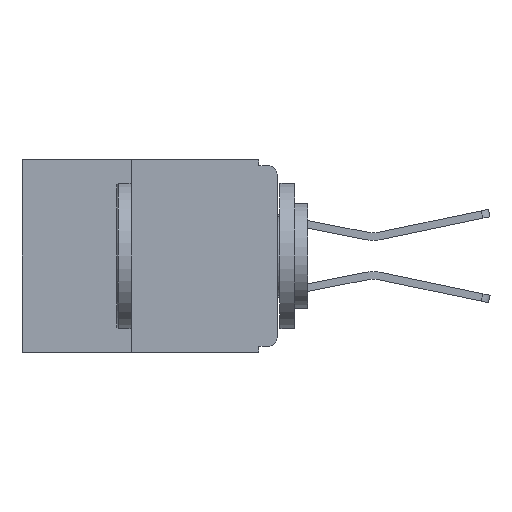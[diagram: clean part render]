
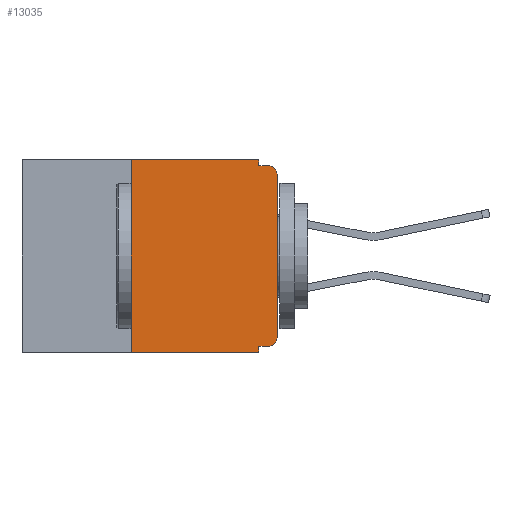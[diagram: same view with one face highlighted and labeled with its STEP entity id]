
A CAD part, left-side view. The second image highlights one B-rep face of the part: STEP entity #13035.
In plain terms, the highlighted planar face has unit normal (-1, 0, 0).
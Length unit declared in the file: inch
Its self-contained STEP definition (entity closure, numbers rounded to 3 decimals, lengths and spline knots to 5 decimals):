
#142 = LINE ( 'NONE', #11878, #17876 ) ;
#284 = PLANE ( 'NONE',  #6104 ) ;
#497 = LINE ( 'NONE', #16744, #20799 ) ;
#806 = VECTOR ( 'NONE', #19617, 39.37008 ) ;
#1842 = EDGE_CURVE ( 'NONE', #16972, #13826, #2128, .T. ) ;
#2007 = DIRECTION ( 'NONE',  ( 0., 1., 0. ) ) ;
#2038 = DIRECTION ( 'NONE',  ( 0., 0., -1. ) ) ;
#2128 = CIRCLE ( 'NONE', #12743, 0.015 ) ;
#2918 = CARTESIAN_POINT ( 'NONE',  ( 0., 0.437, -0.33 ) ) ;
#3091 = EDGE_LOOP ( 'NONE', ( #5953, #6841, #7279, #8026, #8221, #8850, #8959, #9410, #9436, #9678 ) ) ;
#3708 = EDGE_CURVE ( 'NONE', #13333, #16972, #19767, .T. ) ;
#3955 = FACE_OUTER_BOUND ( 'NONE', #3091, .T. ) ;
#4401 = VECTOR ( 'NONE', #7815, 39.37008 ) ;
#5539 = LINE ( 'NONE', #18326, #6081 ) ;
#5917 = EDGE_CURVE ( 'NONE', #13370, #14967, #497, .T. ) ;
#5953 = ORIENTED_EDGE ( 'NONE', *, *, #3708, .T. ) ;
#6081 = VECTOR ( 'NONE', #7314, 39.37008 ) ;
#6104 = AXIS2_PLACEMENT_3D ( 'NONE', #7017, #11906, #2038 ) ;
#6739 = CARTESIAN_POINT ( 'NONE',  ( 0., 0.015, -0.32 ) ) ;
#6783 = CARTESIAN_POINT ( 'NONE',  ( 0., 0.031, 0. ) ) ;
#6839 = CARTESIAN_POINT ( 'NONE',  ( 0., 0.015, -0.305 ) ) ;
#6841 = ORIENTED_EDGE ( 'NONE', *, *, #1842, .T. ) ;
#7017 = CARTESIAN_POINT ( 'NONE',  ( 0., 0.437, 0. ) ) ;
#7279 = ORIENTED_EDGE ( 'NONE', *, *, #15990, .F. ) ;
#7314 = DIRECTION ( 'NONE',  ( 0., 0., 1. ) ) ;
#7450 = EDGE_CURVE ( 'NONE', #12885, #13370, #142, .T. ) ;
#7681 = EDGE_CURVE ( 'NONE', #9169, #18396, #13587, .T. ) ;
#7815 = DIRECTION ( 'NONE',  ( 0., 0., -1. ) ) ;
#8026 = ORIENTED_EDGE ( 'NONE', *, *, #7681, .F. ) ;
#8184 = CARTESIAN_POINT ( 'NONE',  ( 0., 0.031, -0.32 ) ) ;
#8221 = ORIENTED_EDGE ( 'NONE', *, *, #17126, .F. ) ;
#8466 = DIRECTION ( 'NONE',  ( 0., 0., -1. ) ) ;
#8850 = ORIENTED_EDGE ( 'NONE', *, *, #12443, .F. ) ;
#8959 = ORIENTED_EDGE ( 'NONE', *, *, #10276, .T. ) ;
#9169 = VERTEX_POINT ( 'NONE', #6783 ) ;
#9184 = LINE ( 'NONE', #18092, #806 ) ;
#9410 = ORIENTED_EDGE ( 'NONE', *, *, #5917, .F. ) ;
#9436 = ORIENTED_EDGE ( 'NONE', *, *, #7450, .F. ) ;
#9678 = ORIENTED_EDGE ( 'NONE', *, *, #15358, .T. ) ;
#10170 = DIRECTION ( 'NONE',  ( 0., 0., -1. ) ) ;
#10276 = EDGE_CURVE ( 'NONE', #13499, #14967, #13769, .T. ) ;
#11878 = CARTESIAN_POINT ( 'NONE',  ( 0., 0., -0.32 ) ) ;
#11906 = DIRECTION ( 'NONE',  ( 1., 0., 0. ) ) ;
#12387 = VERTEX_POINT ( 'NONE', #13677 ) ;
#12443 = EDGE_CURVE ( 'NONE', #13499, #12387, #5539, .T. ) ;
#12738 = DIRECTION ( 'NONE',  ( 0., -1., 0. ) ) ;
#12743 = AXIS2_PLACEMENT_3D ( 'NONE', #20575, #19091, #10170 ) ;
#12885 = VERTEX_POINT ( 'NONE', #6739 ) ;
#13035 = ADVANCED_FACE ( 'NONE', ( #3955 ), #284, .F. ) ;
#13261 = VECTOR ( 'NONE', #12738, 39.37008 ) ;
#13333 = VERTEX_POINT ( 'NONE', #19001 ) ;
#13370 = VERTEX_POINT ( 'NONE', #8184 ) ;
#13499 = VERTEX_POINT ( 'NONE', #19460 ) ;
#13587 = LINE ( 'NONE', #18803, #4401 ) ;
#13677 = CARTESIAN_POINT ( 'NONE',  ( 0., 0.25, 0. ) ) ;
#13769 = LINE ( 'NONE', #2918, #13261 ) ;
#13826 = VERTEX_POINT ( 'NONE', #18784 ) ;
#14967 = VERTEX_POINT ( 'NONE', #15327 ) ;
#15327 = CARTESIAN_POINT ( 'NONE',  ( 0., 0.031, -0.33 ) ) ;
#15358 = EDGE_CURVE ( 'NONE', #12885, #13333, #16205, .T. ) ;
#15990 = EDGE_CURVE ( 'NONE', #18396, #13826, #16426, .T. ) ;
#16205 = CIRCLE ( 'NONE', #20205, 0.015 ) ;
#16249 = CARTESIAN_POINT ( 'NONE',  ( 0., 0., -0.025 ) ) ;
#16258 = DIRECTION ( 'NONE',  ( 0., 0., 1. ) ) ;
#16359 = CARTESIAN_POINT ( 'NONE',  ( 0., 0., 0. ) ) ;
#16426 = LINE ( 'NONE', #16479, #20436 ) ;
#16479 = CARTESIAN_POINT ( 'NONE',  ( 0., 0., -0.01 ) ) ;
#16682 = DIRECTION ( 'NONE',  ( 0., 0., -1. ) ) ;
#16744 = CARTESIAN_POINT ( 'NONE',  ( 0., 0.031, -0.33 ) ) ;
#16972 = VERTEX_POINT ( 'NONE', #16249 ) ;
#17126 = EDGE_CURVE ( 'NONE', #12387, #9169, #9184, .T. ) ;
#17857 = DIRECTION ( 'NONE',  ( -1., 0., 0. ) ) ;
#17876 = VECTOR ( 'NONE', #2007, 39.37008 ) ;
#18092 = CARTESIAN_POINT ( 'NONE',  ( 0., 0.437, 0. ) ) ;
#18326 = CARTESIAN_POINT ( 'NONE',  ( 0., 0.25, -0.33 ) ) ;
#18396 = VERTEX_POINT ( 'NONE', #19975 ) ;
#18784 = CARTESIAN_POINT ( 'NONE',  ( 0., 0.015, -0.01 ) ) ;
#18803 = CARTESIAN_POINT ( 'NONE',  ( 0., 0.031, 0. ) ) ;
#19001 = CARTESIAN_POINT ( 'NONE',  ( 0., 0., -0.305 ) ) ;
#19091 = DIRECTION ( 'NONE',  ( -1., 0., 0. ) ) ;
#19282 = VECTOR ( 'NONE', #16258, 39.37008 ) ;
#19460 = CARTESIAN_POINT ( 'NONE',  ( 0., 0.25, -0.33 ) ) ;
#19502 = DIRECTION ( 'NONE',  ( 0., -1., 0. ) ) ;
#19617 = DIRECTION ( 'NONE',  ( 0., -1., 0. ) ) ;
#19767 = LINE ( 'NONE', #16359, #19282 ) ;
#19975 = CARTESIAN_POINT ( 'NONE',  ( 0., 0.031, -0.01 ) ) ;
#20205 = AXIS2_PLACEMENT_3D ( 'NONE', #6839, #17857, #8466 ) ;
#20436 = VECTOR ( 'NONE', #19502, 39.37008 ) ;
#20575 = CARTESIAN_POINT ( 'NONE',  ( 0., 0.015, -0.025 ) ) ;
#20799 = VECTOR ( 'NONE', #16682, 39.37008 ) ;
